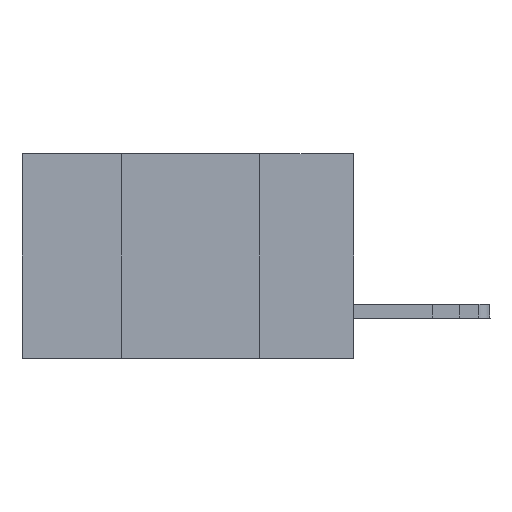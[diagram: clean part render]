
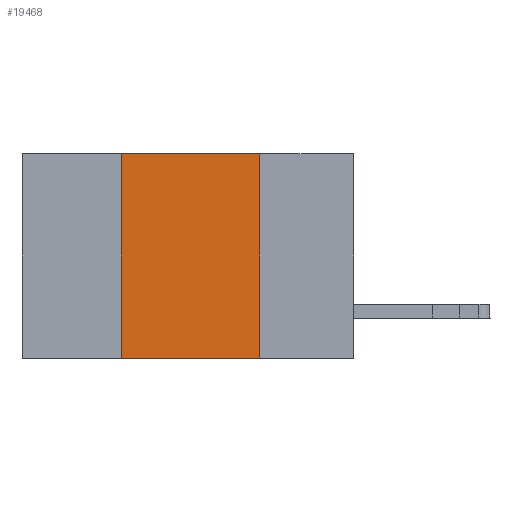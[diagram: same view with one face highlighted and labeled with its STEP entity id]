
A CAD part, left-side view. The second image highlights one B-rep face of the part: STEP entity #19468.
In plain terms, the highlighted planar face has unit normal (-1, 0, 0).
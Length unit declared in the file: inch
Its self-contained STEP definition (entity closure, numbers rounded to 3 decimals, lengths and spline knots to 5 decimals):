
#415 = EDGE_LOOP ( 'NONE', ( #4104, #9174, #14854, #17724 ) ) ;
#1870 = DIRECTION ( 'NONE',  ( 0., -1., 0. ) ) ;
#3300 = VERTEX_POINT ( 'NONE', #9326 ) ;
#4104 = ORIENTED_EDGE ( 'NONE', *, *, #8079, .F. ) ;
#6281 = DIRECTION ( 'NONE',  ( 0., 0., 1. ) ) ;
#6652 = CARTESIAN_POINT ( 'NONE',  ( 0., 0.6, 0. ) ) ;
#7761 = CARTESIAN_POINT ( 'NONE',  ( 0., 0.42, 0. ) ) ;
#8079 = EDGE_CURVE ( 'NONE', #19659, #3300, #12041, .T. ) ;
#8553 = DIRECTION ( 'NONE',  ( 0., 0., -1. ) ) ;
#8717 = FACE_OUTER_BOUND ( 'NONE', #415, .T. ) ;
#8749 = VERTEX_POINT ( 'NONE', #9811 ) ;
#9046 = LINE ( 'NONE', #7761, #14096 ) ;
#9174 = ORIENTED_EDGE ( 'NONE', *, *, #12953, .F. ) ;
#9326 = CARTESIAN_POINT ( 'NONE',  ( 0., 0.17, -0.37 ) ) ;
#9811 = CARTESIAN_POINT ( 'NONE',  ( 0., 0.42, 0. ) ) ;
#10703 = CARTESIAN_POINT ( 'NONE',  ( 0., 0.17, 0. ) ) ;
#11463 = CARTESIAN_POINT ( 'NONE',  ( 0., 0.42, -0.37 ) ) ;
#12041 = LINE ( 'NONE', #10703, #18745 ) ;
#12096 = AXIS2_PLACEMENT_3D ( 'NONE', #17782, #17712, #8553 ) ;
#12953 = EDGE_CURVE ( 'NONE', #8749, #19659, #18056, .T. ) ;
#12975 = CARTESIAN_POINT ( 'NONE',  ( 0., 0.6, -0.37 ) ) ;
#13039 = VECTOR ( 'NONE', #1870, 39.37008 ) ;
#13126 = PLANE ( 'NONE',  #12096 ) ;
#13833 = DIRECTION ( 'NONE',  ( 0., 0., -1. ) ) ;
#14096 = VECTOR ( 'NONE', #6281, 39.37008 ) ;
#14293 = VECTOR ( 'NONE', #16033, 39.37008 ) ;
#14854 = ORIENTED_EDGE ( 'NONE', *, *, #17353, .F. ) ;
#15574 = VERTEX_POINT ( 'NONE', #11463 ) ;
#16033 = DIRECTION ( 'NONE',  ( 0., -1., 0. ) ) ;
#17151 = LINE ( 'NONE', #12975, #14293 ) ;
#17353 = EDGE_CURVE ( 'NONE', #15574, #8749, #9046, .T. ) ;
#17712 = DIRECTION ( 'NONE',  ( 1., 0., 0. ) ) ;
#17724 = ORIENTED_EDGE ( 'NONE', *, *, #18257, .T. ) ;
#17782 = CARTESIAN_POINT ( 'NONE',  ( 0., 0.6, 0. ) ) ;
#18056 = LINE ( 'NONE', #6652, #13039 ) ;
#18257 = EDGE_CURVE ( 'NONE', #15574, #3300, #17151, .T. ) ;
#18745 = VECTOR ( 'NONE', #13833, 39.37008 ) ;
#19468 = ADVANCED_FACE ( 'NONE', ( #8717 ), #13126, .F. ) ;
#19659 = VERTEX_POINT ( 'NONE', #19686 ) ;
#19686 = CARTESIAN_POINT ( 'NONE',  ( 0., 0.17, 0. ) ) ;
